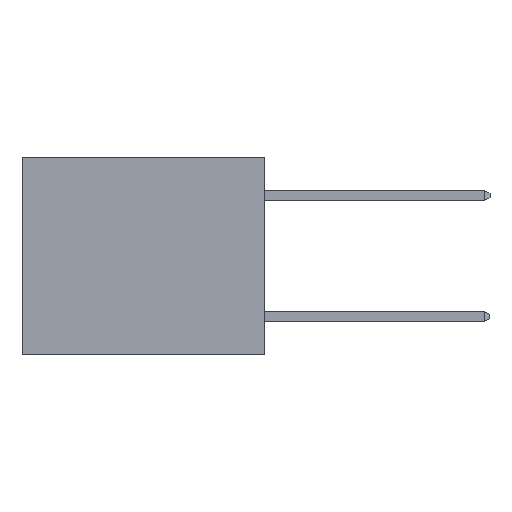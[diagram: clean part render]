
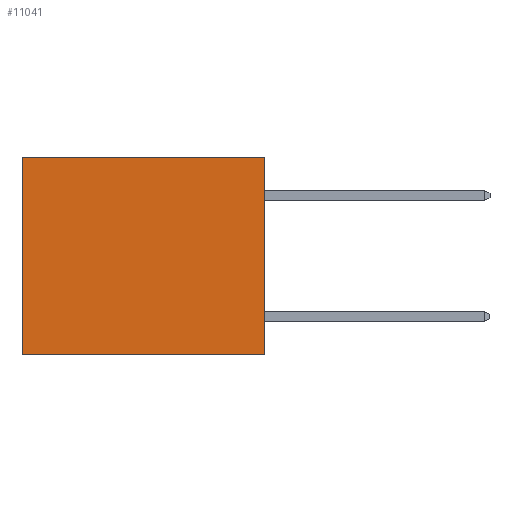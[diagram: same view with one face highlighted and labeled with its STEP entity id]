
A CAD part, left-side view. The second image highlights one B-rep face of the part: STEP entity #11041.
In plain terms, the highlighted planar face has unit normal (-1, 0, 0).
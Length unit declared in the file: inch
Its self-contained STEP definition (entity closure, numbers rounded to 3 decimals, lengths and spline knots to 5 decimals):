
#165 = CARTESIAN_POINT ( 'NONE',  ( 0.3165, 0., -0.49 ) ) ;
#332 = EDGE_CURVE ( 'NONE', #11234, #5901, #5165, .T. ) ;
#1438 = CARTESIAN_POINT ( 'NONE',  ( 0.3165, 0.6, -0.49 ) ) ;
#1587 = CARTESIAN_POINT ( 'NONE',  ( 0.3165, 0., 0. ) ) ;
#2237 = DIRECTION ( 'NONE',  ( 0., 0., -1. ) ) ;
#2474 = VECTOR ( 'NONE', #3984, 39.37008 ) ;
#2800 = LINE ( 'NONE', #9093, #6258 ) ;
#3114 = FACE_OUTER_BOUND ( 'NONE', #7944, .T. ) ;
#3539 = ORIENTED_EDGE ( 'NONE', *, *, #4466, .T. ) ;
#3984 = DIRECTION ( 'NONE',  ( 0., 0., -1. ) ) ;
#4106 = CARTESIAN_POINT ( 'NONE',  ( 0.3165, 0.6, 0. ) ) ;
#4457 = VERTEX_POINT ( 'NONE', #4106 ) ;
#4466 = EDGE_CURVE ( 'NONE', #4457, #5901, #6956, .T. ) ;
#5165 = LINE ( 'NONE', #9296, #7979 ) ;
#5415 = DIRECTION ( 'NONE',  ( 0., 1., 0. ) ) ;
#5901 = VERTEX_POINT ( 'NONE', #1438 ) ;
#5906 = ORIENTED_EDGE ( 'NONE', *, *, #332, .F. ) ;
#5921 = DIRECTION ( 'NONE',  ( 1., 0., 0. ) ) ;
#6119 = CARTESIAN_POINT ( 'NONE',  ( 0.3165, 0., 0. ) ) ;
#6258 = VECTOR ( 'NONE', #8069, 39.37008 ) ;
#6450 = ORIENTED_EDGE ( 'NONE', *, *, #11205, .T. ) ;
#6775 = VERTEX_POINT ( 'NONE', #6119 ) ;
#6953 = PLANE ( 'NONE',  #7789 ) ;
#6956 = LINE ( 'NONE', #11654, #2474 ) ;
#7789 = AXIS2_PLACEMENT_3D ( 'NONE', #165, #5921, #2237 ) ;
#7944 = EDGE_LOOP ( 'NONE', ( #3539, #5906, #9686, #6450 ) ) ;
#7979 = VECTOR ( 'NONE', #12164, 39.37008 ) ;
#8069 = DIRECTION ( 'NONE',  ( 0., 0., -1. ) ) ;
#8275 = CARTESIAN_POINT ( 'NONE',  ( 0.3165, 0., -0.49 ) ) ;
#9093 = CARTESIAN_POINT ( 'NONE',  ( 0.3165, 0., -0.49 ) ) ;
#9296 = CARTESIAN_POINT ( 'NONE',  ( 0.3165, 0., -0.49 ) ) ;
#9686 = ORIENTED_EDGE ( 'NONE', *, *, #11113, .F. ) ;
#10427 = VECTOR ( 'NONE', #5415, 39.37008 ) ;
#11041 = ADVANCED_FACE ( 'NONE', ( #3114 ), #6953, .F. ) ;
#11113 = EDGE_CURVE ( 'NONE', #6775, #11234, #2800, .T. ) ;
#11205 = EDGE_CURVE ( 'NONE', #6775, #4457, #12360, .T. ) ;
#11234 = VERTEX_POINT ( 'NONE', #8275 ) ;
#11654 = CARTESIAN_POINT ( 'NONE',  ( 0.3165, 0.6, -0.49 ) ) ;
#12164 = DIRECTION ( 'NONE',  ( 0., 1., 0. ) ) ;
#12360 = LINE ( 'NONE', #1587, #10427 ) ;
